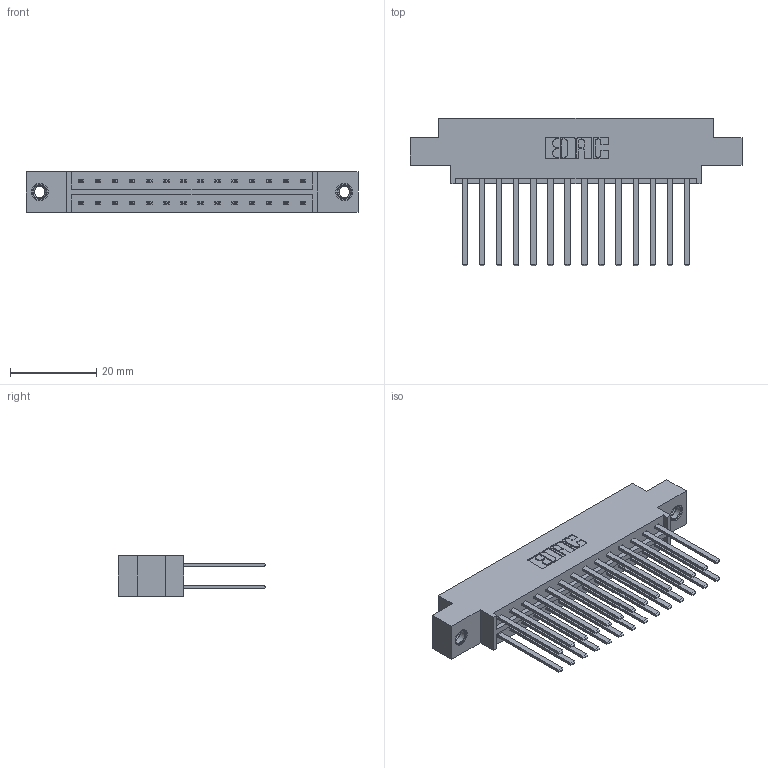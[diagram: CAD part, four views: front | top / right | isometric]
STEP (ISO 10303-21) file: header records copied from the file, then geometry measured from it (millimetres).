
FILE_DESCRIPTION (( 'STEP AP203' ), '1' );
FILE_NAME ('833-028-544-807.STEP', '2020-06-02T09:26:30', ( '' ), ( '' ), 'SwSTEP 2.0', 'SolidWorks 2020', '' );
FILE_SCHEMA (( 'CONFIG_CONTROL_DESIGN' ));
Length unit declared in the file: inch
Products named in the file (4): 345-292-001_345-293-144; 345-250-001_345-250-005-103; 833 Part_Offset - .156 Dia - TI; 833-028-544-807
Assembly tree (31 placements, depth 2):
  833-028-544-807
    833 Part_Offset - .156 Dia - TI
    345-292-001_345-293-144  x28
    345-250-001_345-250-005-103  x2
Bounding box: 77.01 x 34.3 x 9.4 mm (x, y, z)
Volume: 7751.9 mm3; surface area: 10382.6 mm2
Topology: 31 solids, 31 shells, 1466 faces, 4295 edges, 2818 vertices
Faces by surface type: plane 1002, cylinder 448, cone 12, torus 4
Entity records: 13762 total; most frequent: CARTESIAN_POINT 2297, ORIENTED_EDGE 2226, DIRECTION 2039, EDGE_CURVE 1113, LINE 969, VECTOR 969, VERTEX_POINT 736, AXIS2_PLACEMENT_3D 535
